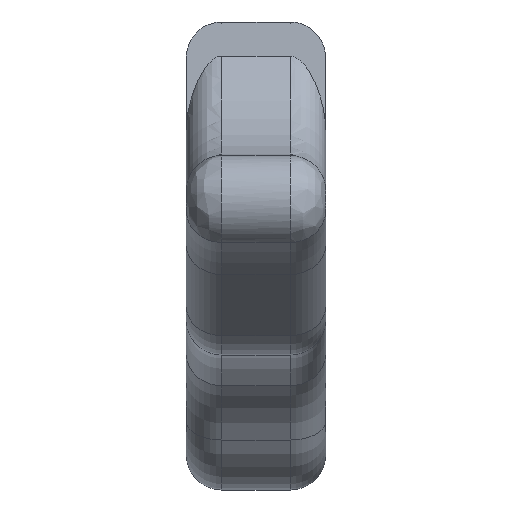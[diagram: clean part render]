
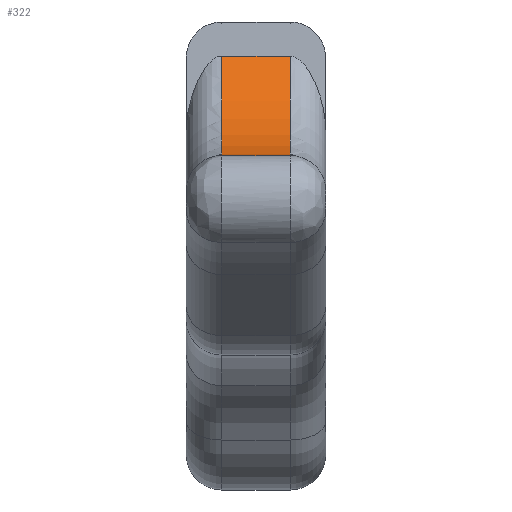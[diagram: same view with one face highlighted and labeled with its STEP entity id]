
A CAD part, front view. The second image highlights one B-rep face of the part: STEP entity #322.
In plain terms, the highlighted cylindrical face has radius 12.652 mm (diameter 25.304 mm), a partial arc.
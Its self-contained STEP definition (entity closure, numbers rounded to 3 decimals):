
#32 = AXIS2_PLACEMENT_3D ( 'NONE', #2764, #874, #3071 ) ;
#194 = DIRECTION ( 'NONE',  ( 0., 0., -1. ) ) ;
#322 = ADVANCED_FACE ( 'NONE', ( #2182 ), #3138, .F. ) ;
#498 = LINE ( 'NONE', #3664, #2305 ) ;
#516 = EDGE_CURVE ( 'NONE', #906, #950, #2554, .T. ) ;
#564 = ORIENTED_EDGE ( 'NONE', *, *, #516, .T. ) ;
#644 = CIRCLE ( 'NONE', #32, 12.652 ) ;
#695 = DIRECTION ( 'NONE',  ( 1., 0., 0. ) ) ;
#874 = DIRECTION ( 'NONE',  ( 1., 0., 0. ) ) ;
#906 = VERTEX_POINT ( 'NONE', #3208 ) ;
#950 = VERTEX_POINT ( 'NONE', #1385 ) ;
#1362 = CARTESIAN_POINT ( 'NONE',  ( -2.398, -9.625, 18.978 ) ) ;
#1385 = CARTESIAN_POINT ( 'NONE',  ( 2.398, -8.853, 6.35 ) ) ;
#1478 = DIRECTION ( 'NONE',  ( 1., 0., 0. ) ) ;
#1589 = CARTESIAN_POINT ( 'NONE',  ( 2.398, 1.777, 13.495 ) ) ;
#1689 = DIRECTION ( 'NONE',  ( 0., 0., -1. ) ) ;
#1900 = ORIENTED_EDGE ( 'NONE', *, *, #2186, .F. ) ;
#1996 = VERTEX_POINT ( 'NONE', #3329 ) ;
#2182 = FACE_OUTER_BOUND ( 'NONE', #3104, .T. ) ;
#2184 = CIRCLE ( 'NONE', #2926, 12.652 ) ;
#2186 = EDGE_CURVE ( 'NONE', #1996, #3080, #498, .T. ) ;
#2262 = AXIS2_PLACEMENT_3D ( 'NONE', #2416, #2307, #194 ) ;
#2280 = CARTESIAN_POINT ( 'NONE',  ( -26.013, -8.853, 6.35 ) ) ;
#2305 = VECTOR ( 'NONE', #1478, 1000. ) ;
#2307 = DIRECTION ( 'NONE',  ( 1., 0., 0. ) ) ;
#2416 = CARTESIAN_POINT ( 'NONE',  ( -26.013, -9.625, 18.978 ) ) ;
#2523 = VECTOR ( 'NONE', #695, 1000. ) ;
#2554 = LINE ( 'NONE', #2280, #2523 ) ;
#2643 = ORIENTED_EDGE ( 'NONE', *, *, #3202, .T. ) ;
#2749 = ORIENTED_EDGE ( 'NONE', *, *, #3655, .T. ) ;
#2764 = CARTESIAN_POINT ( 'NONE',  ( 2.398, -9.625, 18.978 ) ) ;
#2926 = AXIS2_PLACEMENT_3D ( 'NONE', #1362, #3549, #1689 ) ;
#3071 = DIRECTION ( 'NONE',  ( 0., 0., -1. ) ) ;
#3080 = VERTEX_POINT ( 'NONE', #1589 ) ;
#3104 = EDGE_LOOP ( 'NONE', ( #564, #2749, #1900, #2643 ) ) ;
#3138 = CYLINDRICAL_SURFACE ( 'NONE', #2262, 12.652 ) ;
#3202 = EDGE_CURVE ( 'NONE', #1996, #906, #2184, .T. ) ;
#3208 = CARTESIAN_POINT ( 'NONE',  ( -2.398, -8.853, 6.35 ) ) ;
#3329 = CARTESIAN_POINT ( 'NONE',  ( -2.398, 1.777, 13.495 ) ) ;
#3549 = DIRECTION ( 'NONE',  ( -1., 0., 0. ) ) ;
#3655 = EDGE_CURVE ( 'NONE', #950, #3080, #644, .T. ) ;
#3664 = CARTESIAN_POINT ( 'NONE',  ( -26.013, 1.777, 13.495 ) ) ;
